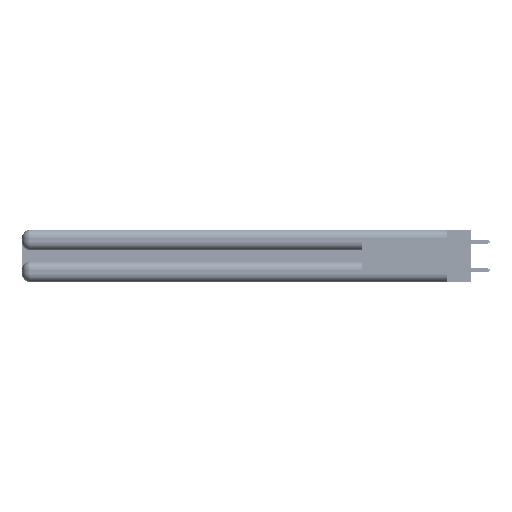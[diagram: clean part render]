
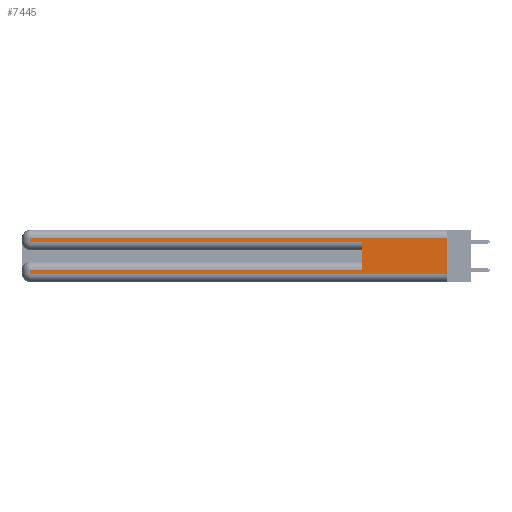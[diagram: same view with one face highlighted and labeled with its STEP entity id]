
A CAD part, left-side view. The second image highlights one B-rep face of the part: STEP entity #7445.
In plain terms, the highlighted planar face has unit normal (-1, 0, 0).
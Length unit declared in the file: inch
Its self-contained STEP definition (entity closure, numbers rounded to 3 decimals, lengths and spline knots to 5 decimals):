
#1805 = LINE ( 'NONE', #8162, #9254 ) ;
#4162 = CARTESIAN_POINT ( 'NONE',  ( 0., 2.94, 0.37 ) ) ;
#4316 = CARTESIAN_POINT ( 'NONE',  ( 0., 0., 0.06 ) ) ;
#4382 = VERTEX_POINT ( 'NONE', #8597 ) ;
#4448 = ORIENTED_EDGE ( 'NONE', *, *, #17288, .F. ) ;
#6142 = DIRECTION ( 'NONE',  ( 0., 0., -1. ) ) ;
#7445 = ADVANCED_FACE ( 'NONE', ( #26251 ), #53476, .F. ) ;
#8162 = CARTESIAN_POINT ( 'NONE',  ( 0., 2.94, 0.37 ) ) ;
#8349 = EDGE_CURVE ( 'NONE', #12615, #17124, #55760, .T. ) ;
#8365 = EDGE_CURVE ( 'NONE', #47154, #20418, #1805, .T. ) ;
#8597 = CARTESIAN_POINT ( 'NONE',  ( 0., 0., 0.06 ) ) ;
#9254 = VECTOR ( 'NONE', #42455, 39.37008 ) ;
#10436 = EDGE_CURVE ( 'NONE', #12615, #22905, #31295, .T. ) ;
#11877 = ORIENTED_EDGE ( 'NONE', *, *, #53788, .T. ) ;
#12419 = EDGE_CURVE ( 'NONE', #44055, #47154, #53343, .T. ) ;
#12605 = CARTESIAN_POINT ( 'NONE',  ( 0., 0., 0.31 ) ) ;
#12615 = VERTEX_POINT ( 'NONE', #32232 ) ;
#12637 = DIRECTION ( 'NONE',  ( 0., -1., 0. ) ) ;
#13926 = ORIENTED_EDGE ( 'NONE', *, *, #12419, .T. ) ;
#14436 = VERTEX_POINT ( 'NONE', #21140 ) ;
#17124 = VERTEX_POINT ( 'NONE', #30022 ) ;
#17288 = EDGE_CURVE ( 'NONE', #44055, #4382, #49050, .T. ) ;
#17568 = DIRECTION ( 'NONE',  ( 0., 0., -1. ) ) ;
#17748 = ORIENTED_EDGE ( 'NONE', *, *, #8349, .F. ) ;
#17840 = VECTOR ( 'NONE', #12637, 39.37008 ) ;
#20418 = VERTEX_POINT ( 'NONE', #53799 ) ;
#20734 = VECTOR ( 'NONE', #25148, 39.37008 ) ;
#21140 = CARTESIAN_POINT ( 'NONE',  ( 0., 2.94, 0.06 ) ) ;
#22905 = VERTEX_POINT ( 'NONE', #34465 ) ;
#23387 = CARTESIAN_POINT ( 'NONE',  ( 0., 2.94, 0.31 ) ) ;
#24869 = DIRECTION ( 'NONE',  ( 0., 1., 0. ) ) ;
#25148 = DIRECTION ( 'NONE',  ( 0., 0., 1. ) ) ;
#26034 = CARTESIAN_POINT ( 'NONE',  ( 0., 0., 0.31 ) ) ;
#26251 = FACE_OUTER_BOUND ( 'NONE', #52099, .T. ) ;
#26348 = ORIENTED_EDGE ( 'NONE', *, *, #10436, .T. ) ;
#27677 = CARTESIAN_POINT ( 'NONE',  ( 0., 0., 0.37 ) ) ;
#28213 = ORIENTED_EDGE ( 'NONE', *, *, #8365, .T. ) ;
#30022 = CARTESIAN_POINT ( 'NONE',  ( 0., 0.6, 0.285 ) ) ;
#30147 = VECTOR ( 'NONE', #38658, 39.37008 ) ;
#31026 = VECTOR ( 'NONE', #32085, 39.37008 ) ;
#31295 = LINE ( 'NONE', #42017, #42716 ) ;
#31322 = LINE ( 'NONE', #4316, #17840 ) ;
#32085 = DIRECTION ( 'NONE',  ( 0., -1., 0. ) ) ;
#32232 = CARTESIAN_POINT ( 'NONE',  ( 0., 0.6, 0.085 ) ) ;
#34465 = CARTESIAN_POINT ( 'NONE',  ( 0., 2.94, 0.085 ) ) ;
#34485 = VECTOR ( 'NONE', #24869, 39.37008 ) ;
#34537 = CARTESIAN_POINT ( 'NONE',  ( 0., 0., 0.37 ) ) ;
#37659 = EDGE_CURVE ( 'NONE', #14436, #4382, #31322, .T. ) ;
#38243 = AXIS2_PLACEMENT_3D ( 'NONE', #27677, #45345, #6142 ) ;
#38658 = DIRECTION ( 'NONE',  ( 0., 0., -1. ) ) ;
#42017 = CARTESIAN_POINT ( 'NONE',  ( 0., 0., 0.085 ) ) ;
#42455 = DIRECTION ( 'NONE',  ( 0., 0., -1. ) ) ;
#42716 = VECTOR ( 'NONE', #46681, 39.37008 ) ;
#44055 = VERTEX_POINT ( 'NONE', #12605 ) ;
#45345 = DIRECTION ( 'NONE',  ( 1., 0., 0. ) ) ;
#46681 = DIRECTION ( 'NONE',  ( 0., 1., 0. ) ) ;
#46898 = EDGE_CURVE ( 'NONE', #22905, #14436, #53059, .T. ) ;
#47112 = CARTESIAN_POINT ( 'NONE',  ( 0., 0.6, 0.145 ) ) ;
#47154 = VERTEX_POINT ( 'NONE', #23387 ) ;
#47794 = LINE ( 'NONE', #49907, #31026 ) ;
#49050 = LINE ( 'NONE', #34537, #52430 ) ;
#49907 = CARTESIAN_POINT ( 'NONE',  ( 0., 0., 0.285 ) ) ;
#51519 = ORIENTED_EDGE ( 'NONE', *, *, #46898, .T. ) ;
#52099 = EDGE_LOOP ( 'NONE', ( #4448, #13926, #28213, #11877, #17748, #26348, #51519, #54104 ) ) ;
#52430 = VECTOR ( 'NONE', #17568, 39.37008 ) ;
#53059 = LINE ( 'NONE', #4162, #30147 ) ;
#53343 = LINE ( 'NONE', #26034, #34485 ) ;
#53476 = PLANE ( 'NONE',  #38243 ) ;
#53788 = EDGE_CURVE ( 'NONE', #20418, #17124, #47794, .T. ) ;
#53799 = CARTESIAN_POINT ( 'NONE',  ( 0., 2.94, 0.285 ) ) ;
#54104 = ORIENTED_EDGE ( 'NONE', *, *, #37659, .T. ) ;
#55760 = LINE ( 'NONE', #47112, #20734 ) ;
